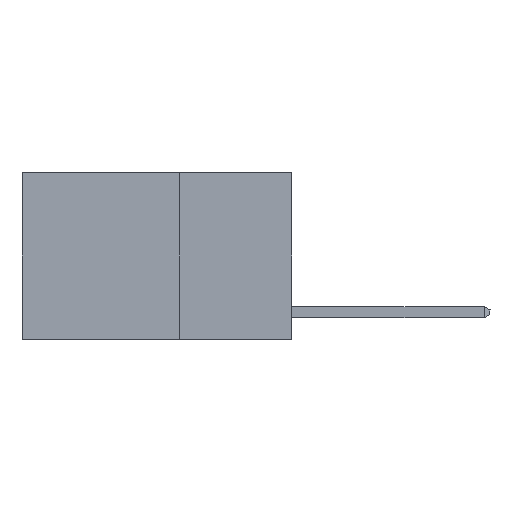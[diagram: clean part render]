
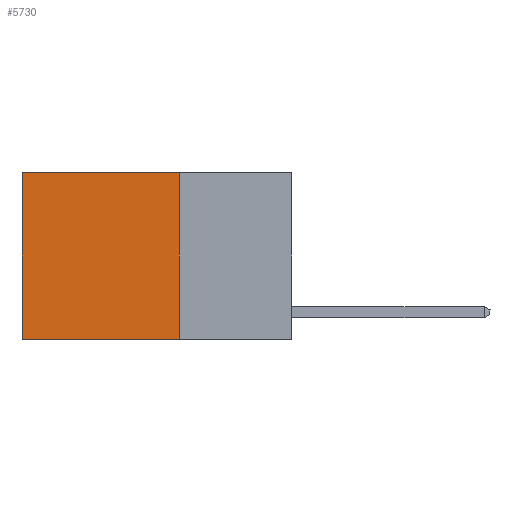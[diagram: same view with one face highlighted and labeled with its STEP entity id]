
A CAD part, left-side view. The second image highlights one B-rep face of the part: STEP entity #5730.
In plain terms, the highlighted planar face has unit normal (-1, 0, 0).
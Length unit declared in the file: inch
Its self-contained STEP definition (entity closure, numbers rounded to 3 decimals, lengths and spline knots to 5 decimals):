
#435 = VECTOR ( 'NONE', #13125, 39.37008 ) ;
#909 = LINE ( 'NONE', #20444, #20404 ) ;
#1018 = LINE ( 'NONE', #11286, #435 ) ;
#2060 = ORIENTED_EDGE ( 'NONE', *, *, #14437, .T. ) ;
#4254 = CARTESIAN_POINT ( 'NONE',  ( 0.2625, 0.6, -0.37 ) ) ;
#4400 = AXIS2_PLACEMENT_3D ( 'NONE', #18036, #7109, #19863 ) ;
#4717 = FACE_OUTER_BOUND ( 'NONE', #13398, .T. ) ;
#5730 = ADVANCED_FACE ( 'NONE', ( #4717 ), #14389, .F. ) ;
#5984 = DIRECTION ( 'NONE',  ( 0., 1., 0. ) ) ;
#6025 = DIRECTION ( 'NONE',  ( 0., 1., 0. ) ) ;
#6706 = VERTEX_POINT ( 'NONE', #4254 ) ;
#7109 = DIRECTION ( 'NONE',  ( 1., 0., 0. ) ) ;
#7749 = CARTESIAN_POINT ( 'NONE',  ( 0.2625, 0.25, 0. ) ) ;
#7785 = DIRECTION ( 'NONE',  ( 0., 0., -1. ) ) ;
#7806 = ORIENTED_EDGE ( 'NONE', *, *, #19690, .T. ) ;
#11286 = CARTESIAN_POINT ( 'NONE',  ( 0.2625, 0.25, 0. ) ) ;
#11894 = CARTESIAN_POINT ( 'NONE',  ( 0.2625, 0.6, 0. ) ) ;
#13125 = DIRECTION ( 'NONE',  ( 0., 0., -1. ) ) ;
#13249 = ORIENTED_EDGE ( 'NONE', *, *, #22602, .F. ) ;
#13398 = EDGE_LOOP ( 'NONE', ( #7806, #13249, #20281, #2060 ) ) ;
#13752 = VERTEX_POINT ( 'NONE', #11894 ) ;
#13846 = CARTESIAN_POINT ( 'NONE',  ( 0.2625, 0.25, -0.37 ) ) ;
#14389 = PLANE ( 'NONE',  #4400 ) ;
#14437 = EDGE_CURVE ( 'NONE', #20125, #13752, #22103, .T. ) ;
#15007 = CARTESIAN_POINT ( 'NONE',  ( 0.2625, 0.25, 0. ) ) ;
#16840 = EDGE_CURVE ( 'NONE', #20125, #22850, #1018, .T. ) ;
#17318 = VECTOR ( 'NONE', #5984, 39.37008 ) ;
#18036 = CARTESIAN_POINT ( 'NONE',  ( 0.2625, 0.25, 0. ) ) ;
#19690 = EDGE_CURVE ( 'NONE', #13752, #6706, #909, .T. ) ;
#19863 = DIRECTION ( 'NONE',  ( 0., 0., -1. ) ) ;
#20125 = VERTEX_POINT ( 'NONE', #15007 ) ;
#20281 = ORIENTED_EDGE ( 'NONE', *, *, #16840, .F. ) ;
#20404 = VECTOR ( 'NONE', #7785, 39.37008 ) ;
#20444 = CARTESIAN_POINT ( 'NONE',  ( 0.2625, 0.6, 0. ) ) ;
#20611 = CARTESIAN_POINT ( 'NONE',  ( 0.2625, 0.25, -0.37 ) ) ;
#21377 = VECTOR ( 'NONE', #6025, 39.37008 ) ;
#21919 = LINE ( 'NONE', #20611, #21377 ) ;
#22103 = LINE ( 'NONE', #7749, #17318 ) ;
#22602 = EDGE_CURVE ( 'NONE', #22850, #6706, #21919, .T. ) ;
#22850 = VERTEX_POINT ( 'NONE', #13846 ) ;
